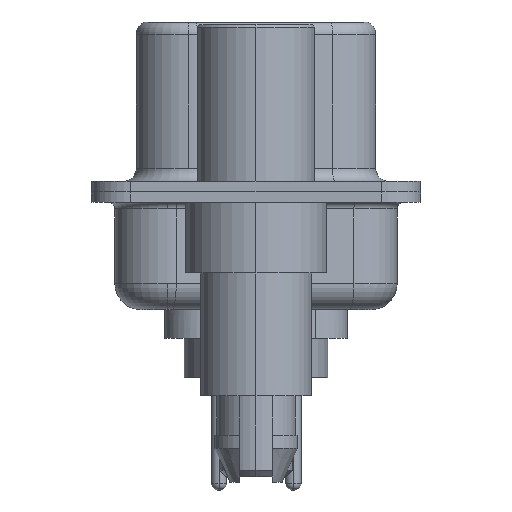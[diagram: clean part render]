
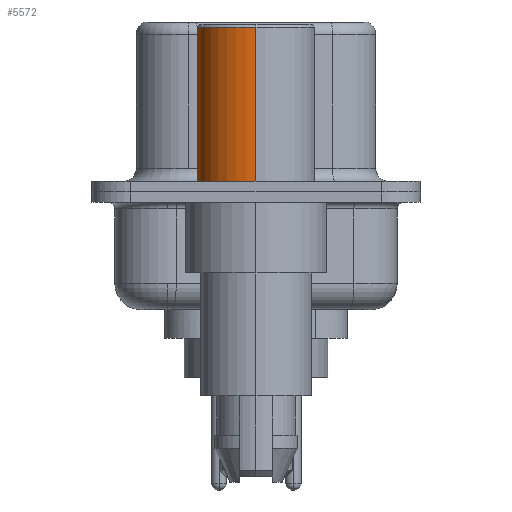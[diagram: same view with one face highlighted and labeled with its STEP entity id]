
A CAD part, left-side view. The second image highlights one B-rep face of the part: STEP entity #5572.
In plain terms, the highlighted cylindrical face has radius 2.25 mm (diameter 4.5 mm), a partial arc.
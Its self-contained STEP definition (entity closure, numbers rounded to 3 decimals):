
#622 = DIRECTION ( 'NONE',  ( 1., 0., 0. ) ) ;
#755 = CIRCLE ( 'NONE', #14434, 2.25 ) ;
#1287 = ORIENTED_EDGE ( 'NONE', *, *, #7912, .F. ) ;
#1693 = CARTESIAN_POINT ( 'NONE',  ( 2.25, 0., 0.581 ) ) ;
#1934 = AXIS2_PLACEMENT_3D ( 'NONE', #3677, #2491, #14666 ) ;
#2126 = CARTESIAN_POINT ( 'NONE',  ( 0., 0., 6.3 ) ) ;
#2491 = DIRECTION ( 'NONE',  ( 0., 0., 1. ) ) ;
#2551 = FACE_OUTER_BOUND ( 'NONE', #8511, .T. ) ;
#2817 = ORIENTED_EDGE ( 'NONE', *, *, #8004, .T. ) ;
#2894 = DIRECTION ( 'NONE',  ( 0., 0., 1. ) ) ;
#2993 = DIRECTION ( 'NONE',  ( 0., 0., 1. ) ) ;
#3358 = DIRECTION ( 'NONE',  ( 1., 0., 0. ) ) ;
#3629 = LINE ( 'NONE', #1693, #6976 ) ;
#3677 = CARTESIAN_POINT ( 'NONE',  ( 0., 0., 0.581 ) ) ;
#4976 = CIRCLE ( 'NONE', #8412, 2.25 ) ;
#5284 = VERTEX_POINT ( 'NONE', #10203 ) ;
#5572 = ADVANCED_FACE ( 'NONE', ( #2551 ), #12029, .T. ) ;
#6191 = VECTOR ( 'NONE', #2993, 1000. ) ;
#6244 = ORIENTED_EDGE ( 'NONE', *, *, #8030, .T. ) ;
#6327 = VERTEX_POINT ( 'NONE', #15874 ) ;
#6976 = VECTOR ( 'NONE', #2894, 1000. ) ;
#7708 = ORIENTED_EDGE ( 'NONE', *, *, #8161, .F. ) ;
#7912 = EDGE_CURVE ( 'NONE', #15678, #5284, #3629, .T. ) ;
#8004 = EDGE_CURVE ( 'NONE', #13937, #6327, #9487, .T. ) ;
#8030 = EDGE_CURVE ( 'NONE', #15678, #13937, #755, .T. ) ;
#8054 = DIRECTION ( 'NONE',  ( 0., 0., 1. ) ) ;
#8161 = EDGE_CURVE ( 'NONE', #5284, #6327, #4976, .T. ) ;
#8412 = AXIS2_PLACEMENT_3D ( 'NONE', #2126, #10819, #3358 ) ;
#8511 = EDGE_LOOP ( 'NONE', ( #6244, #2817, #7708, #1287 ) ) ;
#9163 = CARTESIAN_POINT ( 'NONE',  ( -2.25, 0., 0.581 ) ) ;
#9487 = LINE ( 'NONE', #9163, #6191 ) ;
#10203 = CARTESIAN_POINT ( 'NONE',  ( 2.25, 0., 6.3 ) ) ;
#10819 = DIRECTION ( 'NONE',  ( 0., 0., 1. ) ) ;
#12029 = CYLINDRICAL_SURFACE ( 'NONE', #1934, 2.25 ) ;
#13686 = CARTESIAN_POINT ( 'NONE',  ( 2.25, 0., 0.4 ) ) ;
#13937 = VERTEX_POINT ( 'NONE', #15416 ) ;
#14434 = AXIS2_PLACEMENT_3D ( 'NONE', #15380, #8054, #622 ) ;
#14666 = DIRECTION ( 'NONE',  ( 1., 0., 0. ) ) ;
#15380 = CARTESIAN_POINT ( 'NONE',  ( 0., 0., 0.4 ) ) ;
#15416 = CARTESIAN_POINT ( 'NONE',  ( -2.25, 0., 0.4 ) ) ;
#15678 = VERTEX_POINT ( 'NONE', #13686 ) ;
#15874 = CARTESIAN_POINT ( 'NONE',  ( -2.25, 0., 6.3 ) ) ;
